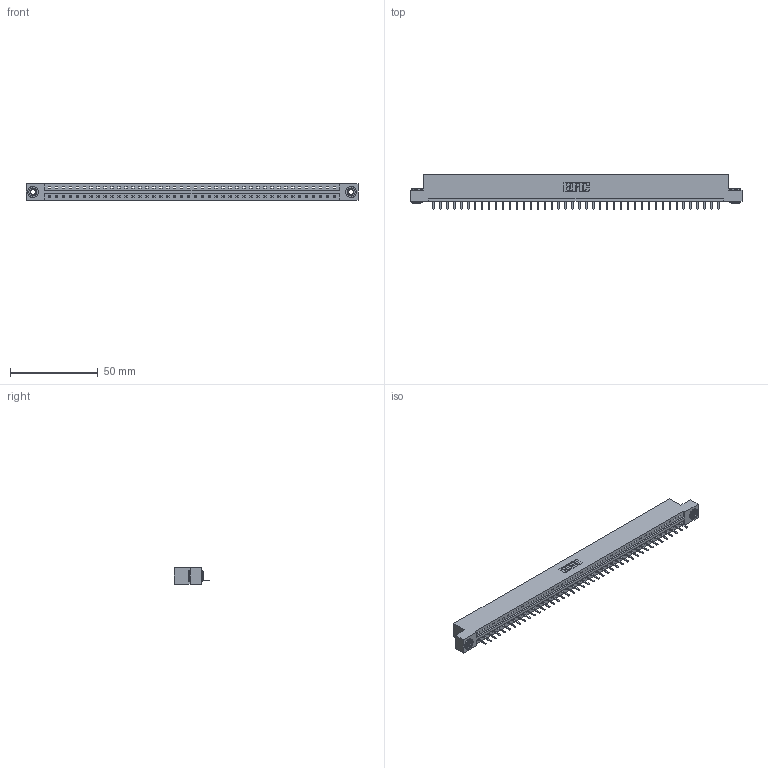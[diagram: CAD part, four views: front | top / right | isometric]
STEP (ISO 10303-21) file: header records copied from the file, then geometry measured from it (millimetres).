
FILE_DESCRIPTION (( 'STEP AP203' ), '1' );
FILE_NAME ('337-042-520-103.STEP', '2018-08-08T22:55:56', ( '' ), ( '' ), 'SwSTEP 2.0', 'SolidWorks 2016', '' );
FILE_SCHEMA (( 'CONFIG_CONTROL_DESIGN' ));
Length unit declared in the file: inch
Products named in the file (4): 337 Part_Flush Mounting Lugs - 0.156 Dia-TH; 345-292-001_345-293-120; 345-250-002_345-250-002-102; 337-042-520-103
Assembly tree (45 placements, depth 2):
  337-042-520-103
    337 Part_Flush Mounting Lugs - 0.156 Dia-TH
    345-292-001_345-293-120  x42
    345-250-002_345-250-002-102  x2
Bounding box: 189.43 x 20.02 x 9.4 mm (x, y, z)
Volume: 19587 mm3; surface area: 20038.1 mm2
Topology: 45 solids, 45 shells, 2924 faces, 8619 edges, 5630 vertices
Faces by surface type: plane 2096, cylinder 820, cone 8
Entity records: 31984 total; most frequent: CARTESIAN_POINT 5559, ORIENTED_EDGE 5518, DIRECTION 4701, EDGE_CURVE 2759, VECTOR 2603, LINE 2603, VERTEX_POINT 1834, AXIS2_PLACEMENT_3D 1049
